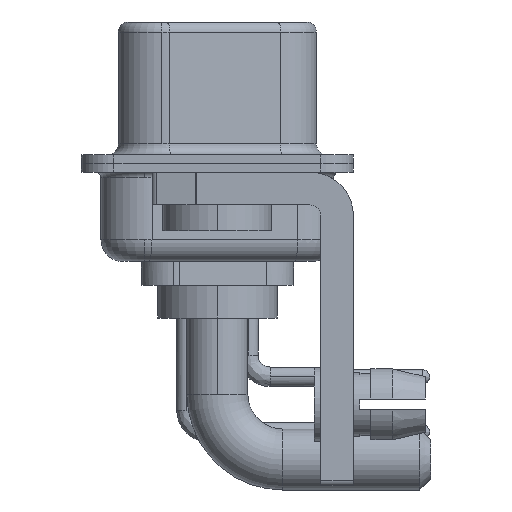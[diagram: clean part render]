
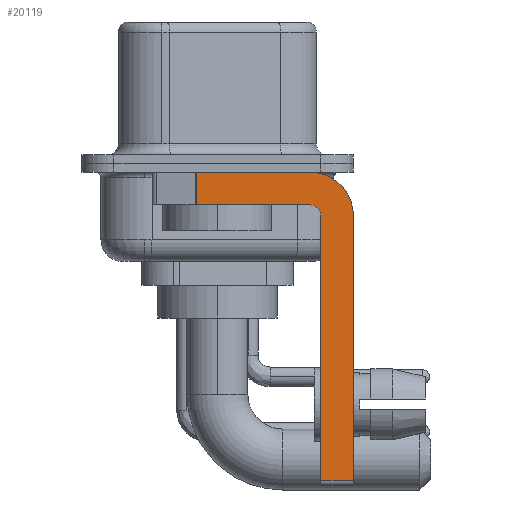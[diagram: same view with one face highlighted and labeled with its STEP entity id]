
A CAD part, left-side view. The second image highlights one B-rep face of the part: STEP entity #20119.
In plain terms, the highlighted planar face has unit normal (-1, 0, 0).
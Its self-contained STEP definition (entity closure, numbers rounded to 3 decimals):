
#169 = VECTOR ( 'NONE', #20954, 1000. ) ;
#441 = VECTOR ( 'NONE', #12088, 1000. ) ;
#837 = CARTESIAN_POINT ( 'NONE',  ( -2.9, 3., -0.4 ) ) ;
#936 = ORIENTED_EDGE ( 'NONE', *, *, #11506, .T. ) ;
#1763 = VERTEX_POINT ( 'NONE', #17161 ) ;
#1915 = EDGE_CURVE ( 'NONE', #1763, #18345, #25762, .T. ) ;
#2071 = DIRECTION ( 'NONE',  ( 0., 0., 1. ) ) ;
#3032 = EDGE_CURVE ( 'NONE', #3998, #20284, #25287, .T. ) ;
#3211 = VECTOR ( 'NONE', #17022, 1000. ) ;
#3414 = VERTEX_POINT ( 'NONE', #15175 ) ;
#3483 = AXIS2_PLACEMENT_3D ( 'NONE', #22449, #18745, #2071 ) ;
#3998 = VERTEX_POINT ( 'NONE', #13702 ) ;
#4034 = LINE ( 'NONE', #6018, #441 ) ;
#4784 = LINE ( 'NONE', #4909, #24164 ) ;
#4909 = CARTESIAN_POINT ( 'NONE',  ( -2.9, -4.25, -1.9 ) ) ;
#5093 = ORIENTED_EDGE ( 'NONE', *, *, #22299, .F. ) ;
#5972 = CARTESIAN_POINT ( 'NONE',  ( -2.9, -4.25, -0.4 ) ) ;
#6018 = CARTESIAN_POINT ( 'NONE',  ( -2.9, -4.25, -14.55 ) ) ;
#6333 = ORIENTED_EDGE ( 'NONE', *, *, #21594, .F. ) ;
#6585 = DIRECTION ( 'NONE',  ( 0., 0., -1. ) ) ;
#6772 = LINE ( 'NONE', #837, #169 ) ;
#7372 = VECTOR ( 'NONE', #23301, 1000. ) ;
#7606 = DIRECTION ( 'NONE',  ( 0., 0., -1. ) ) ;
#7621 = VERTEX_POINT ( 'NONE', #25284 ) ;
#8239 = CARTESIAN_POINT ( 'NONE',  ( -2.9, -6.25, -14.55 ) ) ;
#8280 = VECTOR ( 'NONE', #7606, 1000. ) ;
#8754 = ORIENTED_EDGE ( 'NONE', *, *, #14860, .F. ) ;
#8786 = EDGE_CURVE ( 'NONE', #7621, #23977, #4784, .T. ) ;
#9582 = VERTEX_POINT ( 'NONE', #5972 ) ;
#9886 = ORIENTED_EDGE ( 'NONE', *, *, #1915, .F. ) ;
#11054 = DIRECTION ( 'NONE',  ( 1., 0., 0. ) ) ;
#11506 = EDGE_CURVE ( 'NONE', #3998, #18345, #4034, .T. ) ;
#12088 = DIRECTION ( 'NONE',  ( 0., -1., 0. ) ) ;
#12776 = LINE ( 'NONE', #20607, #3211 ) ;
#12843 = DIRECTION ( 'NONE',  ( 0., 1., 0. ) ) ;
#13702 = CARTESIAN_POINT ( 'NONE',  ( -2.9, -4.75, -14.55 ) ) ;
#14044 = DIRECTION ( 'NONE',  ( 1., 0., 0. ) ) ;
#14178 = FACE_OUTER_BOUND ( 'NONE', #22742, .T. ) ;
#14860 = EDGE_CURVE ( 'NONE', #9582, #1763, #16949, .T. ) ;
#14889 = CIRCLE ( 'NONE', #3483, 0.5 ) ;
#15175 = CARTESIAN_POINT ( 'NONE',  ( -2.9, 0.978, -0.4 ) ) ;
#15209 = CARTESIAN_POINT ( 'NONE',  ( -2.9, -4.75, -14.8 ) ) ;
#16949 = CIRCLE ( 'NONE', #21176, 2. ) ;
#17022 = DIRECTION ( 'NONE',  ( 0., 0., -1. ) ) ;
#17161 = CARTESIAN_POINT ( 'NONE',  ( -2.9, -6.25, -2.4 ) ) ;
#18345 = VERTEX_POINT ( 'NONE', #8239 ) ;
#18667 = DIRECTION ( 'NONE',  ( 0., 0., -1. ) ) ;
#18702 = AXIS2_PLACEMENT_3D ( 'NONE', #22383, #14044, #18667 ) ;
#18745 = DIRECTION ( 'NONE',  ( -1., 0., 0. ) ) ;
#19319 = CARTESIAN_POINT ( 'NONE',  ( -2.9, -4.75, -2.4 ) ) ;
#20119 = ADVANCED_FACE ( 'NONE', ( #14178 ), #22650, .F. ) ;
#20273 = CARTESIAN_POINT ( 'NONE',  ( -2.9, 0.978, -1.9 ) ) ;
#20284 = VERTEX_POINT ( 'NONE', #19319 ) ;
#20291 = ORIENTED_EDGE ( 'NONE', *, *, #8786, .F. ) ;
#20607 = CARTESIAN_POINT ( 'NONE',  ( -2.9, 0.978, -1.9 ) ) ;
#20954 = DIRECTION ( 'NONE',  ( 0., -1., 0. ) ) ;
#21176 = AXIS2_PLACEMENT_3D ( 'NONE', #22617, #11054, #6585 ) ;
#21594 = EDGE_CURVE ( 'NONE', #20284, #7621, #14889, .T. ) ;
#22299 = EDGE_CURVE ( 'NONE', #3414, #9582, #6772, .T. ) ;
#22383 = CARTESIAN_POINT ( 'NONE',  ( -2.9, -4.25, -2.4 ) ) ;
#22449 = CARTESIAN_POINT ( 'NONE',  ( -2.9, -4.25, -2.4 ) ) ;
#22617 = CARTESIAN_POINT ( 'NONE',  ( -2.9, -4.25, -2.4 ) ) ;
#22650 = PLANE ( 'NONE',  #18702 ) ;
#22742 = EDGE_LOOP ( 'NONE', ( #5093, #25960, #20291, #6333, #24243, #936, #9886, #8754 ) ) ;
#23301 = DIRECTION ( 'NONE',  ( 0., 0., 1. ) ) ;
#23977 = VERTEX_POINT ( 'NONE', #20273 ) ;
#24164 = VECTOR ( 'NONE', #12843, 1000. ) ;
#24243 = ORIENTED_EDGE ( 'NONE', *, *, #3032, .F. ) ;
#24950 = EDGE_CURVE ( 'NONE', #3414, #23977, #12776, .T. ) ;
#25284 = CARTESIAN_POINT ( 'NONE',  ( -2.9, -4.25, -1.9 ) ) ;
#25287 = LINE ( 'NONE', #15209, #7372 ) ;
#25639 = CARTESIAN_POINT ( 'NONE',  ( -2.9, -6.25, -2.4 ) ) ;
#25762 = LINE ( 'NONE', #25639, #8280 ) ;
#25960 = ORIENTED_EDGE ( 'NONE', *, *, #24950, .T. ) ;
